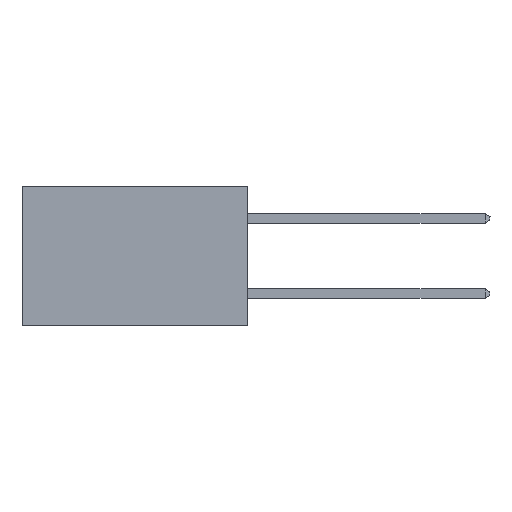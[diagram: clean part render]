
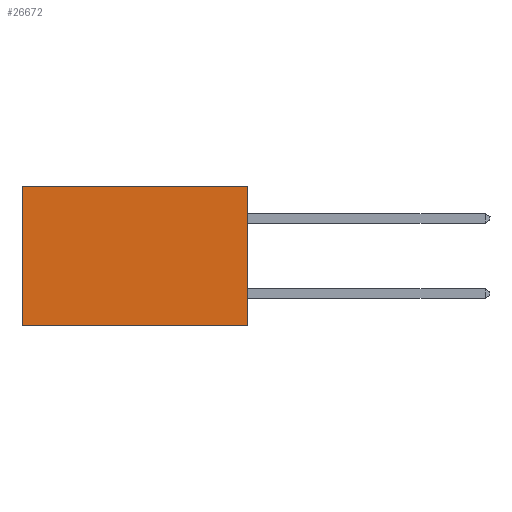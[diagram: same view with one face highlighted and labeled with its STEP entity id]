
A CAD part, left-side view. The second image highlights one B-rep face of the part: STEP entity #26672.
In plain terms, the highlighted planar face has unit normal (-1, 0, 0).
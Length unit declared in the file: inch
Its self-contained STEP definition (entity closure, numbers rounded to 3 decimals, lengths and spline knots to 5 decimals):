
#643 = EDGE_CURVE ( 'NONE', #9448, #16077, #15468, .T. ) ;
#806 = DIRECTION ( 'NONE',  ( 0., 1., 0. ) ) ;
#1783 = CARTESIAN_POINT ( 'NONE',  ( 0.2615, 0.6, 0. ) ) ;
#2457 = CARTESIAN_POINT ( 'NONE',  ( 0.2615, 0., 0. ) ) ;
#3232 = ORIENTED_EDGE ( 'NONE', *, *, #11013, .T. ) ;
#3938 = EDGE_CURVE ( 'NONE', #26843, #9448, #24130, .T. ) ;
#4758 = VERTEX_POINT ( 'NONE', #1783 ) ;
#6373 = CARTESIAN_POINT ( 'NONE',  ( 0.2615, 0.6, -0.37 ) ) ;
#7601 = CARTESIAN_POINT ( 'NONE',  ( 0.2615, 0., -0.37 ) ) ;
#7912 = VECTOR ( 'NONE', #23524, 39.37008 ) ;
#9448 = VERTEX_POINT ( 'NONE', #21546 ) ;
#10034 = ORIENTED_EDGE ( 'NONE', *, *, #3938, .F. ) ;
#11013 = EDGE_CURVE ( 'NONE', #26843, #4758, #19945, .T. ) ;
#11349 = EDGE_CURVE ( 'NONE', #4758, #16077, #22929, .T. ) ;
#11633 = VECTOR ( 'NONE', #806, 39.37008 ) ;
#14074 = CARTESIAN_POINT ( 'NONE',  ( 0.2615, 0.6, -0.37 ) ) ;
#14807 = DIRECTION ( 'NONE',  ( 0., 0., -1. ) ) ;
#15240 = EDGE_LOOP ( 'NONE', ( #20865, #17897, #10034, #3232 ) ) ;
#15468 = LINE ( 'NONE', #17687, #11633 ) ;
#16032 = DIRECTION ( 'NONE',  ( 0., 0., -1. ) ) ;
#16077 = VERTEX_POINT ( 'NONE', #14074 ) ;
#17687 = CARTESIAN_POINT ( 'NONE',  ( 0.2615, 0., -0.37 ) ) ;
#17897 = ORIENTED_EDGE ( 'NONE', *, *, #643, .F. ) ;
#18519 = PLANE ( 'NONE',  #23065 ) ;
#19945 = LINE ( 'NONE', #23661, #7912 ) ;
#20056 = DIRECTION ( 'NONE',  ( 1., 0., 0. ) ) ;
#20865 = ORIENTED_EDGE ( 'NONE', *, *, #11349, .T. ) ;
#21546 = CARTESIAN_POINT ( 'NONE',  ( 0.2615, 0., -0.37 ) ) ;
#22200 = DIRECTION ( 'NONE',  ( 0., 0., -1. ) ) ;
#22468 = CARTESIAN_POINT ( 'NONE',  ( 0.2615, 0., -0.37 ) ) ;
#22929 = LINE ( 'NONE', #6373, #24689 ) ;
#23065 = AXIS2_PLACEMENT_3D ( 'NONE', #7601, #20056, #16032 ) ;
#23524 = DIRECTION ( 'NONE',  ( 0., 1., 0. ) ) ;
#23616 = VECTOR ( 'NONE', #22200, 39.37008 ) ;
#23661 = CARTESIAN_POINT ( 'NONE',  ( 0.2615, 0., 0. ) ) ;
#24130 = LINE ( 'NONE', #22468, #23616 ) ;
#24689 = VECTOR ( 'NONE', #14807, 39.37008 ) ;
#26548 = FACE_OUTER_BOUND ( 'NONE', #15240, .T. ) ;
#26672 = ADVANCED_FACE ( 'NONE', ( #26548 ), #18519, .F. ) ;
#26843 = VERTEX_POINT ( 'NONE', #2457 ) ;
